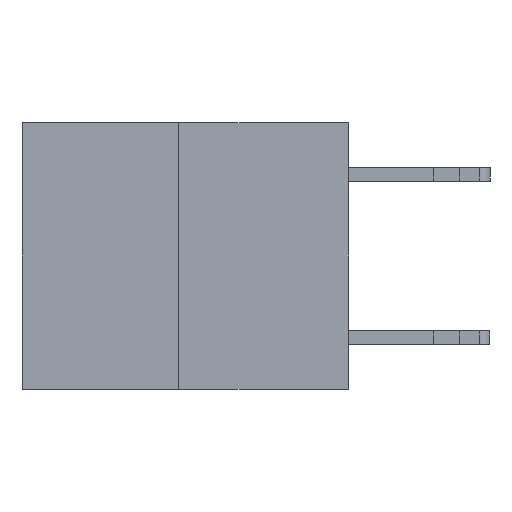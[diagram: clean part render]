
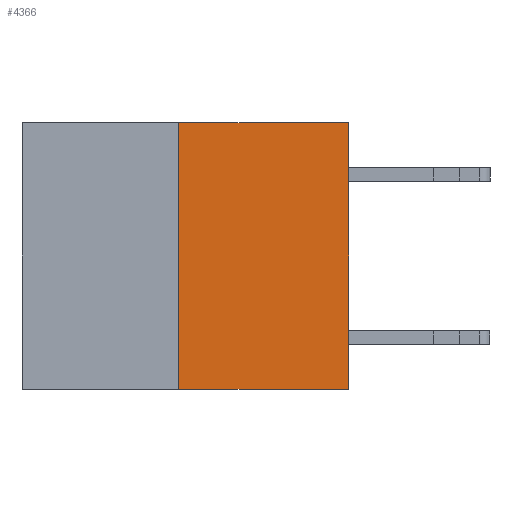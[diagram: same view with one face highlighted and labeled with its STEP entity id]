
A CAD part, left-side view. The second image highlights one B-rep face of the part: STEP entity #4366.
In plain terms, the highlighted planar face has unit normal (-1, 0, 0).
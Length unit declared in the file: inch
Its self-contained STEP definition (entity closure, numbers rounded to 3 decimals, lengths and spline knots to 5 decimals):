
#1306 = LINE ( 'NONE', #18649, #12264 ) ;
#1475 = CARTESIAN_POINT ( 'NONE',  ( 0., 0.6, -0.49 ) ) ;
#1720 = DIRECTION ( 'NONE',  ( 0., -1., 0. ) ) ;
#2758 = VECTOR ( 'NONE', #16571, 39.37008 ) ;
#3155 = DIRECTION ( 'NONE',  ( 0., 0., -1. ) ) ;
#4262 = ORIENTED_EDGE ( 'NONE', *, *, #14982, .T. ) ;
#4366 = ADVANCED_FACE ( 'NONE', ( #18901 ), #19826, .F. ) ;
#4473 = LINE ( 'NONE', #10150, #12550 ) ;
#4678 = VERTEX_POINT ( 'NONE', #19962 ) ;
#4760 = CARTESIAN_POINT ( 'NONE',  ( 0., 0.312, -0.49 ) ) ;
#5638 = VERTEX_POINT ( 'NONE', #14606 ) ;
#5997 = EDGE_CURVE ( 'NONE', #6336, #5638, #6062, .T. ) ;
#6062 = LINE ( 'NONE', #1475, #15922 ) ;
#6336 = VERTEX_POINT ( 'NONE', #4760 ) ;
#6367 = EDGE_CURVE ( 'NONE', #11906, #4678, #4473, .T. ) ;
#6429 = DIRECTION ( 'NONE',  ( 0., -1., 0. ) ) ;
#7053 = ORIENTED_EDGE ( 'NONE', *, *, #18428, .F. ) ;
#7457 = EDGE_LOOP ( 'NONE', ( #7053, #9793, #4262, #11576 ) ) ;
#8094 = CARTESIAN_POINT ( 'NONE',  ( 0., 0.6, 0. ) ) ;
#9793 = ORIENTED_EDGE ( 'NONE', *, *, #5997, .T. ) ;
#10150 = CARTESIAN_POINT ( 'NONE',  ( 0., 0.6, 0. ) ) ;
#11398 = CARTESIAN_POINT ( 'NONE',  ( 0., 0.312, 0. ) ) ;
#11576 = ORIENTED_EDGE ( 'NONE', *, *, #6367, .F. ) ;
#11595 = CARTESIAN_POINT ( 'NONE',  ( 0., 0.312, -0.49 ) ) ;
#11906 = VERTEX_POINT ( 'NONE', #11398 ) ;
#12264 = VECTOR ( 'NONE', #20020, 39.37008 ) ;
#12550 = VECTOR ( 'NONE', #1720, 39.37008 ) ;
#13108 = DIRECTION ( 'NONE',  ( 1., 0., 0. ) ) ;
#13657 = LINE ( 'NONE', #11595, #2758 ) ;
#14606 = CARTESIAN_POINT ( 'NONE',  ( 0., 0., -0.49 ) ) ;
#14982 = EDGE_CURVE ( 'NONE', #5638, #4678, #1306, .T. ) ;
#15922 = VECTOR ( 'NONE', #6429, 39.37008 ) ;
#16571 = DIRECTION ( 'NONE',  ( 0., 0., 1. ) ) ;
#16859 = AXIS2_PLACEMENT_3D ( 'NONE', #8094, #13108, #3155 ) ;
#18428 = EDGE_CURVE ( 'NONE', #6336, #11906, #13657, .T. ) ;
#18649 = CARTESIAN_POINT ( 'NONE',  ( 0., 0., 0. ) ) ;
#18901 = FACE_OUTER_BOUND ( 'NONE', #7457, .T. ) ;
#19826 = PLANE ( 'NONE',  #16859 ) ;
#19962 = CARTESIAN_POINT ( 'NONE',  ( 0., 0., 0. ) ) ;
#20020 = DIRECTION ( 'NONE',  ( 0., 0., 1. ) ) ;
